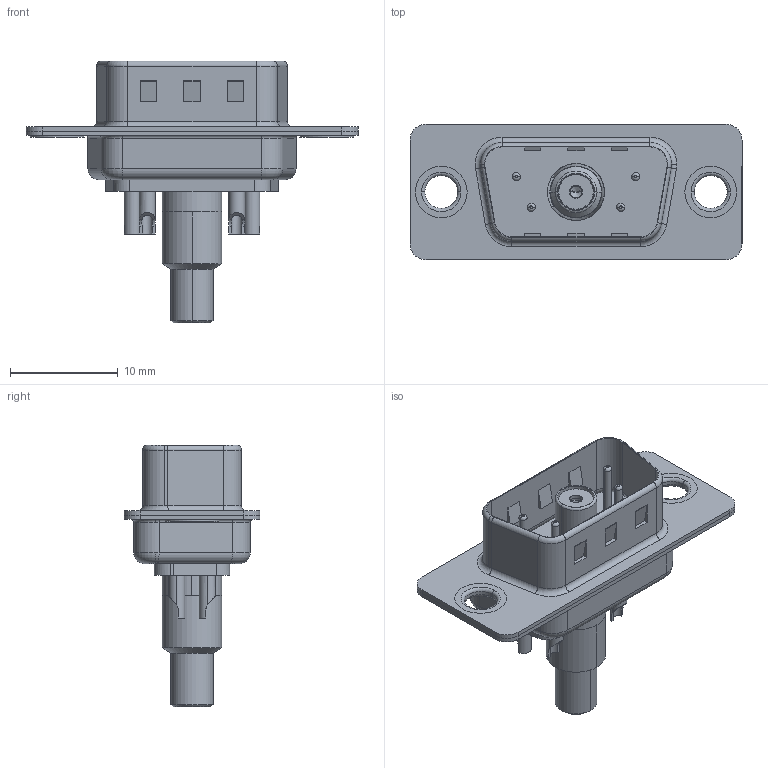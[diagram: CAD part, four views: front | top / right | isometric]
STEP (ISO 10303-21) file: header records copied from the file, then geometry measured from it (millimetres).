
FILE_DESCRIPTION (( 'STEP AP203' ), '1' );
FILE_NAME ('627-5W1-222-5N1.STEP', '2019-05-24T06:34:41', ( '' ), ( '' ), 'SwSTEP 2.0', 'SolidWorks 2016', '' );
FILE_SCHEMA (( 'CONFIG_CONTROL_DESIGN' ));
Length unit declared in the file: millimetre
Products named in the file (14): Co-Ax Jack Assy_SC; 627Combo Shell Front_09 Contacts; 627Combo Contact Row 1_22; 627Combo Thru Hole Rivet; 627Combo Contact Row 2_22; Co-Ax Jack_Solder Cup Tail; 627-5W1-222-5N1; Insulator Socket; Insulator Socket 2; Locking Collar; Socket_Solder Cup; 627Combo Housing_5W1; Solder Cover; 627Combo Shell Rear_09 Contacts
Assembly tree (16 placements, depth 3):
  627-5W1-222-5N1
    627Combo Housing_5W1
    627Combo Shell Rear_09 Contacts
    627Combo Shell Front_09 Contacts
    627Combo Thru Hole Rivet  x2
    Co-Ax Jack Assy_SC
      Co-Ax Jack_Solder Cup Tail
      Insulator Socket
      Insulator Socket 2
      Locking Collar
      Socket_Solder Cup
      Solder Cover
    627Combo Contact Row 1_22  x2
    627Combo Contact Row 2_22  x2
Bounding box: 30.8 x 12.6 x 24.3 mm (x, y, z)
Volume: 1365.6 mm3; surface area: 4271.4 mm2
Topology: 15 solids, 15 shells, 556 faces, 1300 edges, 798 vertices
Faces by surface type: cylinder 241, plane 183, torus 102, cone 28, bspline 2
Entity records: 15549 total; most frequent: DIRECTION 2604, CARTESIAN_POINT 2574, ORIENTED_EDGE 2236, EDGE_CURVE 1118, AXIS2_PLACEMENT_3D 1039, VERTEX_POINT 696, EDGE_LOOP 556, CIRCLE 543
